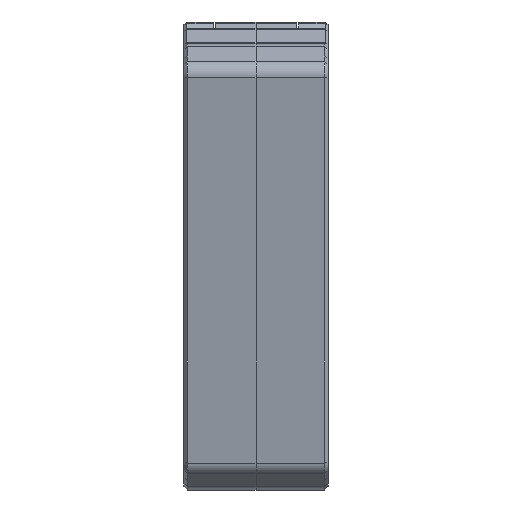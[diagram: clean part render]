
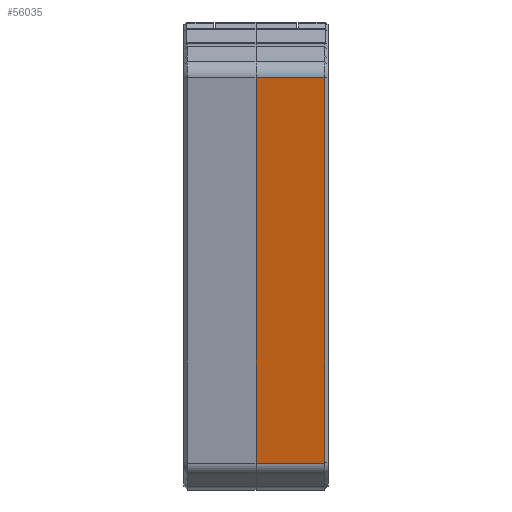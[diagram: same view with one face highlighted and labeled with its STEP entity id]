
A CAD part, front view. The second image highlights one B-rep face of the part: STEP entity #56035.
In plain terms, the highlighted planar face has unit normal (0, -0.983, -0.181).
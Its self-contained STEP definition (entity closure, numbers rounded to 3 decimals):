
#1966 = ORIENTED_EDGE ( 'NONE', *, *, #62247, .F. ) ;
#2182 = EDGE_LOOP ( 'NONE', ( #80590, #39661, #1966, #78238 ) ) ;
#2491 = DIRECTION ( 'NONE',  ( 0., 0.181, -0.983 ) ) ;
#3439 = VECTOR ( 'NONE', #54759, 1000. ) ;
#4014 = CARTESIAN_POINT ( 'NONE',  ( 89.739, -65.815, 32.349 ) ) ;
#5381 = FACE_OUTER_BOUND ( 'NONE', #2182, .T. ) ;
#8660 = LINE ( 'NONE', #29284, #3439 ) ;
#12372 = CARTESIAN_POINT ( 'NONE',  ( 89.739, -53.012, -37.091 ) ) ;
#15877 = CARTESIAN_POINT ( 'NONE',  ( 0., -53.234, -35.889 ) ) ;
#18661 = VERTEX_POINT ( 'NONE', #61690 ) ;
#19553 = EDGE_CURVE ( 'NONE', #43507, #18661, #34913, .T. ) ;
#20448 = VECTOR ( 'NONE', #85269, 1000. ) ;
#24213 = DIRECTION ( 'NONE',  ( 0., 0.181, -0.983 ) ) ;
#28238 = CARTESIAN_POINT ( 'NONE',  ( 12.182, -65.815, 32.349 ) ) ;
#29284 = CARTESIAN_POINT ( 'NONE',  ( 0., -53.012, -37.091 ) ) ;
#34913 = LINE ( 'NONE', #74920, #44783 ) ;
#39661 = ORIENTED_EDGE ( 'NONE', *, *, #58440, .T. ) ;
#43507 = VERTEX_POINT ( 'NONE', #28238 ) ;
#44783 = VECTOR ( 'NONE', #2491, 1000. ) ;
#46136 = LINE ( 'NONE', #59762, #20448 ) ;
#54759 = DIRECTION ( 'NONE',  ( 0., 0.181, -0.983 ) ) ;
#56035 = ADVANCED_FACE ( 'NONE', ( #5381 ), #72539, .T. ) ;
#57714 = VERTEX_POINT ( 'NONE', #15877 ) ;
#58440 = EDGE_CURVE ( 'NONE', #70142, #57714, #8660, .T. ) ;
#59762 = CARTESIAN_POINT ( 'NONE',  ( 89.739, -53.234, -35.889 ) ) ;
#61690 = CARTESIAN_POINT ( 'NONE',  ( 12.182, -53.234, -35.889 ) ) ;
#62247 = EDGE_CURVE ( 'NONE', #18661, #57714, #46136, .T. ) ;
#63359 = AXIS2_PLACEMENT_3D ( 'NONE', #12372, #71226, #24213 ) ;
#70142 = VERTEX_POINT ( 'NONE', #77544 ) ;
#71226 = DIRECTION ( 'NONE',  ( 0., -0.983, -0.181 ) ) ;
#72472 = DIRECTION ( 'NONE',  ( 1., 0., 0. ) ) ;
#72539 = PLANE ( 'NONE',  #63359 ) ;
#74920 = CARTESIAN_POINT ( 'NONE',  ( 12.182, -53.012, -37.091 ) ) ;
#77310 = LINE ( 'NONE', #4014, #86472 ) ;
#77544 = CARTESIAN_POINT ( 'NONE',  ( 0., -65.815, 32.349 ) ) ;
#78238 = ORIENTED_EDGE ( 'NONE', *, *, #19553, .F. ) ;
#80590 = ORIENTED_EDGE ( 'NONE', *, *, #86773, .F. ) ;
#85269 = DIRECTION ( 'NONE',  ( -1., 0., 0. ) ) ;
#86472 = VECTOR ( 'NONE', #72472, 1000. ) ;
#86773 = EDGE_CURVE ( 'NONE', #70142, #43507, #77310, .T. ) ;
